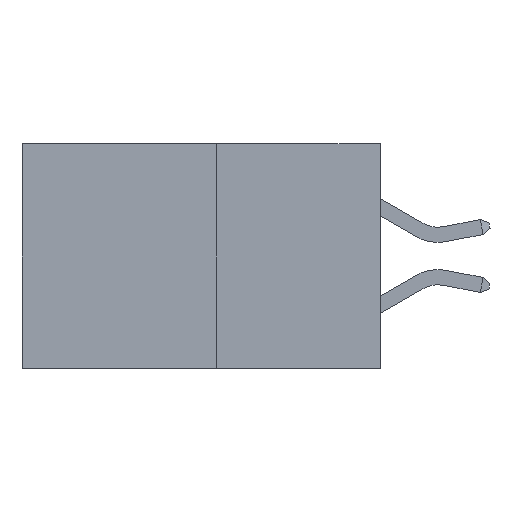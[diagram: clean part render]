
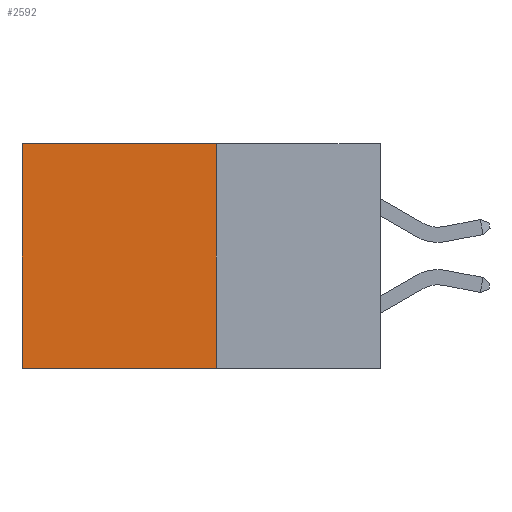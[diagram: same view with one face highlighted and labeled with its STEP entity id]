
A CAD part, left-side view. The second image highlights one B-rep face of the part: STEP entity #2592.
In plain terms, the highlighted planar face has unit normal (-1, 0, 0).
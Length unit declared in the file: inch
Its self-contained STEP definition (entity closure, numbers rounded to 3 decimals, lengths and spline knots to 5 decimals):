
#353 = DIRECTION ( 'NONE',  ( 0., 0., -1. ) ) ;
#589 = VECTOR ( 'NONE', #1590, 39.37008 ) ;
#946 = CARTESIAN_POINT ( 'NONE',  ( 0.277, 0.27, 0. ) ) ;
#1214 = LINE ( 'NONE', #9116, #10626 ) ;
#1542 = ORIENTED_EDGE ( 'NONE', *, *, #18266, .F. ) ;
#1590 = DIRECTION ( 'NONE',  ( 0., 1., 0. ) ) ;
#1639 = CARTESIAN_POINT ( 'NONE',  ( 0.277, 0.27, -0.37 ) ) ;
#2003 = EDGE_LOOP ( 'NONE', ( #7373, #7005, #1542, #15709 ) ) ;
#2592 = ADVANCED_FACE ( 'NONE', ( #7468 ), #12372, .F. ) ;
#2735 = DIRECTION ( 'NONE',  ( 0., 1., 0. ) ) ;
#3178 = AXIS2_PLACEMENT_3D ( 'NONE', #12223, #12219, #12147 ) ;
#4078 = DIRECTION ( 'NONE',  ( 0., 0., -1. ) ) ;
#5381 = LINE ( 'NONE', #946, #18169 ) ;
#6625 = EDGE_CURVE ( 'NONE', #11433, #9585, #19724, .T. ) ;
#6944 = VERTEX_POINT ( 'NONE', #15569 ) ;
#7005 = ORIENTED_EDGE ( 'NONE', *, *, #6625, .F. ) ;
#7373 = ORIENTED_EDGE ( 'NONE', *, *, #19980, .T. ) ;
#7468 = FACE_OUTER_BOUND ( 'NONE', #2003, .T. ) ;
#8033 = CARTESIAN_POINT ( 'NONE',  ( 0.277, 0.27, -0.37 ) ) ;
#9116 = CARTESIAN_POINT ( 'NONE',  ( 0.277, 0.27, -0.37 ) ) ;
#9585 = VERTEX_POINT ( 'NONE', #17334 ) ;
#10626 = VECTOR ( 'NONE', #353, 39.37008 ) ;
#11403 = VERTEX_POINT ( 'NONE', #13121 ) ;
#11433 = VERTEX_POINT ( 'NONE', #8033 ) ;
#12147 = DIRECTION ( 'NONE',  ( 0., 0., -1. ) ) ;
#12219 = DIRECTION ( 'NONE',  ( 1., 0., 0. ) ) ;
#12223 = CARTESIAN_POINT ( 'NONE',  ( 0.277, 0.27, -0.37 ) ) ;
#12372 = PLANE ( 'NONE',  #3178 ) ;
#13121 = CARTESIAN_POINT ( 'NONE',  ( 0.277, 0.59, 0. ) ) ;
#14077 = LINE ( 'NONE', #14582, #14622 ) ;
#14582 = CARTESIAN_POINT ( 'NONE',  ( 0.277, 0.59, -0.37 ) ) ;
#14622 = VECTOR ( 'NONE', #4078, 39.37008 ) ;
#15569 = CARTESIAN_POINT ( 'NONE',  ( 0.277, 0.27, 0. ) ) ;
#15709 = ORIENTED_EDGE ( 'NONE', *, *, #19205, .T. ) ;
#17334 = CARTESIAN_POINT ( 'NONE',  ( 0.277, 0.59, -0.37 ) ) ;
#18169 = VECTOR ( 'NONE', #2735, 39.37008 ) ;
#18266 = EDGE_CURVE ( 'NONE', #6944, #11433, #1214, .T. ) ;
#19205 = EDGE_CURVE ( 'NONE', #6944, #11403, #5381, .T. ) ;
#19724 = LINE ( 'NONE', #1639, #589 ) ;
#19980 = EDGE_CURVE ( 'NONE', #11403, #9585, #14077, .T. ) ;
